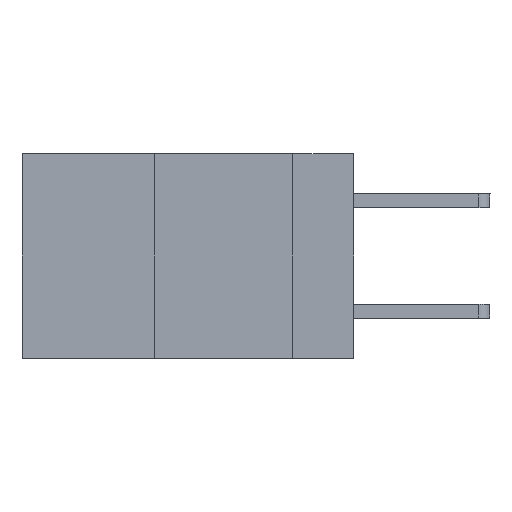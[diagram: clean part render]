
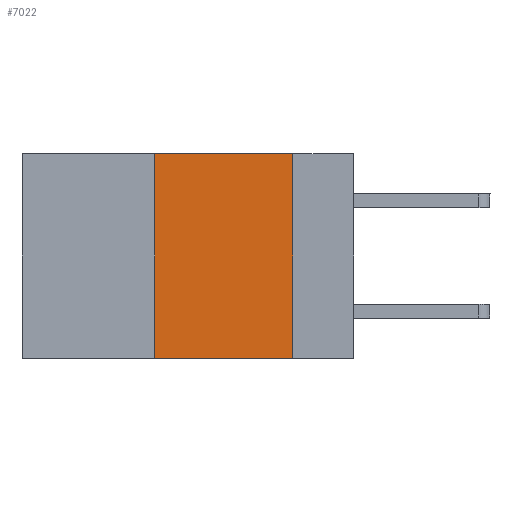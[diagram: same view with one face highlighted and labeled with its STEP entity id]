
A CAD part, left-side view. The second image highlights one B-rep face of the part: STEP entity #7022.
In plain terms, the highlighted planar face has unit normal (-1, 0, 0).
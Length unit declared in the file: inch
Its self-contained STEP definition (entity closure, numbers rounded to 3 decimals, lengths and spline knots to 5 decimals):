
#56 = CARTESIAN_POINT ( 'NONE',  ( 0., 0.11, -0.37 ) ) ;
#66 = CARTESIAN_POINT ( 'NONE',  ( 0., 0.6, 0. ) ) ;
#188 = EDGE_LOOP ( 'NONE', ( #12836, #13768, #13829, #2616 ) ) ;
#202 = VECTOR ( 'NONE', #9756, 39.37008 ) ;
#330 = EDGE_CURVE ( 'NONE', #9057, #5004, #5668, .T. ) ;
#434 = CARTESIAN_POINT ( 'NONE',  ( 0., 0.36, 0. ) ) ;
#593 = LINE ( 'NONE', #10051, #202 ) ;
#794 = LINE ( 'NONE', #5075, #3751 ) ;
#1334 = EDGE_CURVE ( 'NONE', #11050, #11708, #9289, .T. ) ;
#1551 = EDGE_CURVE ( 'NONE', #11708, #9057, #593, .T. ) ;
#1705 = EDGE_CURVE ( 'NONE', #11050, #5004, #794, .T. ) ;
#2616 = ORIENTED_EDGE ( 'NONE', *, *, #1705, .T. ) ;
#2803 = VECTOR ( 'NONE', #11890, 39.37008 ) ;
#2974 = VECTOR ( 'NONE', #6816, 39.37008 ) ;
#3000 = FACE_OUTER_BOUND ( 'NONE', #188, .T. ) ;
#3751 = VECTOR ( 'NONE', #5198, 39.37008 ) ;
#5004 = VERTEX_POINT ( 'NONE', #56 ) ;
#5075 = CARTESIAN_POINT ( 'NONE',  ( 0., 0.6, -0.37 ) ) ;
#5198 = DIRECTION ( 'NONE',  ( 0., -1., 0. ) ) ;
#5511 = CARTESIAN_POINT ( 'NONE',  ( 0., 0.36, 0. ) ) ;
#5668 = LINE ( 'NONE', #10752, #2803 ) ;
#6791 = CARTESIAN_POINT ( 'NONE',  ( 0., 0.36, -0.37 ) ) ;
#6816 = DIRECTION ( 'NONE',  ( 0., 0., 1. ) ) ;
#7022 = ADVANCED_FACE ( 'NONE', ( #3000 ), #9686, .F. ) ;
#7427 = DIRECTION ( 'NONE',  ( 1., 0., 0. ) ) ;
#9057 = VERTEX_POINT ( 'NONE', #14088 ) ;
#9289 = LINE ( 'NONE', #434, #2974 ) ;
#9686 = PLANE ( 'NONE',  #13284 ) ;
#9756 = DIRECTION ( 'NONE',  ( 0., -1., 0. ) ) ;
#10051 = CARTESIAN_POINT ( 'NONE',  ( 0., 0.6, 0. ) ) ;
#10749 = DIRECTION ( 'NONE',  ( 0., 0., -1. ) ) ;
#10752 = CARTESIAN_POINT ( 'NONE',  ( 0., 0.11, 0. ) ) ;
#11050 = VERTEX_POINT ( 'NONE', #6791 ) ;
#11708 = VERTEX_POINT ( 'NONE', #5511 ) ;
#11890 = DIRECTION ( 'NONE',  ( 0., 0., -1. ) ) ;
#12836 = ORIENTED_EDGE ( 'NONE', *, *, #330, .F. ) ;
#13284 = AXIS2_PLACEMENT_3D ( 'NONE', #66, #7427, #10749 ) ;
#13768 = ORIENTED_EDGE ( 'NONE', *, *, #1551, .F. ) ;
#13829 = ORIENTED_EDGE ( 'NONE', *, *, #1334, .F. ) ;
#14088 = CARTESIAN_POINT ( 'NONE',  ( 0., 0.11, 0. ) ) ;
